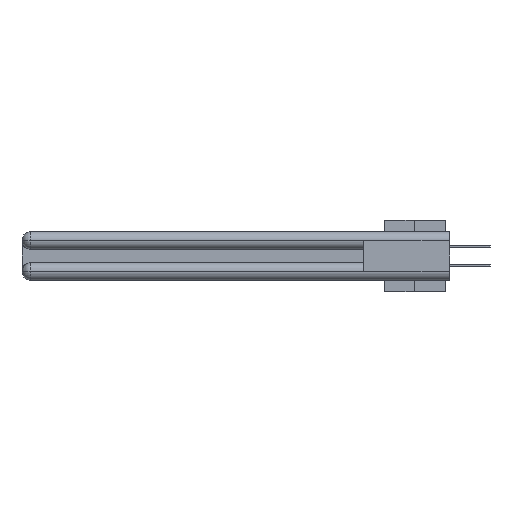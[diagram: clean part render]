
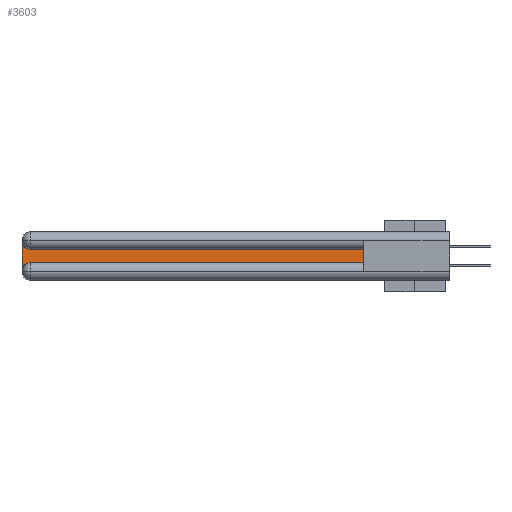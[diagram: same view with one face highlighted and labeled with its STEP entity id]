
A CAD part, left-side view. The second image highlights one B-rep face of the part: STEP entity #3603.
In plain terms, the highlighted planar face has unit normal (-1, 0, 0).
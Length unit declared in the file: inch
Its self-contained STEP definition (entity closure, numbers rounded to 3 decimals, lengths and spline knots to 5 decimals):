
#126 = VECTOR ( 'NONE', #16241, 39.37008 ) ;
#1425 = VERTEX_POINT ( 'NONE', #6501 ) ;
#3603 = ADVANCED_FACE ( 'NONE', ( #8534 ), #40387, .F. ) ;
#3768 = CARTESIAN_POINT ( 'NONE',  ( 0.075, 0.6, -0.1225 ) ) ;
#4529 = CARTESIAN_POINT ( 'NONE',  ( 0.075, 3., -0.1225 ) ) ;
#5186 = VECTOR ( 'NONE', #10464, 39.37008 ) ;
#5486 = EDGE_CURVE ( 'NONE', #22467, #32825, #14468, .T. ) ;
#5854 = ORIENTED_EDGE ( 'NONE', *, *, #8724, .T. ) ;
#6263 = LINE ( 'NONE', #33012, #126 ) ;
#6501 = CARTESIAN_POINT ( 'NONE',  ( 0.075, 3., -0.2775 ) ) ;
#7211 = LINE ( 'NONE', #33100, #5186 ) ;
#8056 = DIRECTION ( 'NONE',  ( 0., 0., -1. ) ) ;
#8534 = FACE_OUTER_BOUND ( 'NONE', #33946, .T. ) ;
#8724 = EDGE_CURVE ( 'NONE', #17623, #31100, #17546, .T. ) ;
#10097 = DIRECTION ( 'NONE',  ( 0., 0., -1. ) ) ;
#10464 = DIRECTION ( 'NONE',  ( 0., -1., 0. ) ) ;
#14045 = DIRECTION ( 'NONE',  ( 1., 0., 0. ) ) ;
#14468 = CIRCLE ( 'NONE', #19742, 0.06 ) ;
#16241 = DIRECTION ( 'NONE',  ( 0., 1., 0. ) ) ;
#16876 = VERTEX_POINT ( 'NONE', #32149 ) ;
#16922 = EDGE_CURVE ( 'NONE', #31100, #22467, #6263, .T. ) ;
#17546 = LINE ( 'NONE', #39010, #29901 ) ;
#17623 = VERTEX_POINT ( 'NONE', #21966 ) ;
#18646 = CARTESIAN_POINT ( 'NONE',  ( 0.075, 3., -0.2175 ) ) ;
#18759 = AXIS2_PLACEMENT_3D ( 'NONE', #19960, #39712, #10097 ) ;
#19162 = ORIENTED_EDGE ( 'NONE', *, *, #5486, .T. ) ;
#19742 = AXIS2_PLACEMENT_3D ( 'NONE', #25960, #29659, #26246 ) ;
#19960 = CARTESIAN_POINT ( 'NONE',  ( 0.075, 2.94, -0.2775 ) ) ;
#20357 = VECTOR ( 'NONE', #28265, 39.37008 ) ;
#21966 = CARTESIAN_POINT ( 'NONE',  ( 0.075, 0.6, -0.2175 ) ) ;
#22467 = VERTEX_POINT ( 'NONE', #39287 ) ;
#23943 = CIRCLE ( 'NONE', #18759, 0.06 ) ;
#24096 = AXIS2_PLACEMENT_3D ( 'NONE', #4529, #14045, #8056 ) ;
#25960 = CARTESIAN_POINT ( 'NONE',  ( 0.075, 2.94, -0.0625 ) ) ;
#26246 = DIRECTION ( 'NONE',  ( 0., 0., -1. ) ) ;
#27656 = EDGE_CURVE ( 'NONE', #32825, #1425, #33196, .T. ) ;
#28265 = DIRECTION ( 'NONE',  ( 0., 0., -1. ) ) ;
#28830 = ORIENTED_EDGE ( 'NONE', *, *, #16922, .T. ) ;
#29659 = DIRECTION ( 'NONE',  ( 1., 0., 0. ) ) ;
#29901 = VECTOR ( 'NONE', #32281, 39.37008 ) ;
#31100 = VERTEX_POINT ( 'NONE', #3768 ) ;
#32149 = CARTESIAN_POINT ( 'NONE',  ( 0.075, 2.94, -0.2175 ) ) ;
#32281 = DIRECTION ( 'NONE',  ( 0., 0., 1. ) ) ;
#32825 = VERTEX_POINT ( 'NONE', #37735 ) ;
#33012 = CARTESIAN_POINT ( 'NONE',  ( 0.075, 0.6, -0.1225 ) ) ;
#33100 = CARTESIAN_POINT ( 'NONE',  ( 0.075, 0.6, -0.2175 ) ) ;
#33196 = LINE ( 'NONE', #18646, #20357 ) ;
#33946 = EDGE_LOOP ( 'NONE', ( #28830, #19162, #39407, #41332, #42062, #5854 ) ) ;
#35460 = EDGE_CURVE ( 'NONE', #16876, #17623, #7211, .T. ) ;
#37735 = CARTESIAN_POINT ( 'NONE',  ( 0.075, 3., -0.0625 ) ) ;
#38140 = EDGE_CURVE ( 'NONE', #1425, #16876, #23943, .T. ) ;
#39010 = CARTESIAN_POINT ( 'NONE',  ( 0.075, 0.6, -0.2175 ) ) ;
#39287 = CARTESIAN_POINT ( 'NONE',  ( 0.075, 2.94, -0.1225 ) ) ;
#39407 = ORIENTED_EDGE ( 'NONE', *, *, #27656, .T. ) ;
#39712 = DIRECTION ( 'NONE',  ( 1., 0., 0. ) ) ;
#40387 = PLANE ( 'NONE',  #24096 ) ;
#41332 = ORIENTED_EDGE ( 'NONE', *, *, #38140, .T. ) ;
#42062 = ORIENTED_EDGE ( 'NONE', *, *, #35460, .T. ) ;
